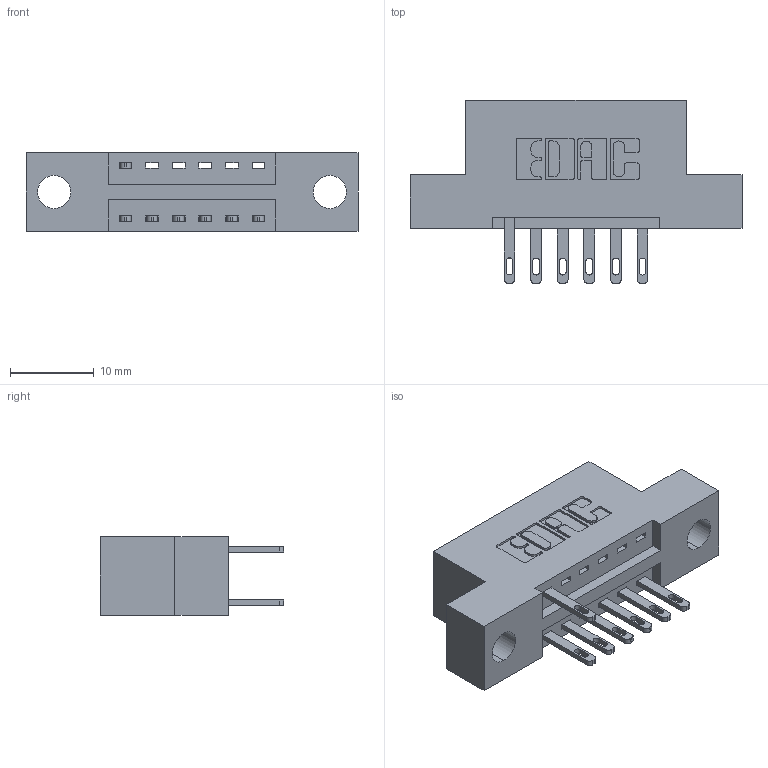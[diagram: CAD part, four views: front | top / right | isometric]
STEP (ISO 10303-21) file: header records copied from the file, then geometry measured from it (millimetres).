
FILE_DESCRIPTION (( 'STEP AP203' ), '1' );
FILE_NAME ('346-012-500-204.STEP', '2018-08-19T21:36:17', ( '' ), ( '' ), 'SwSTEP 2.0', 'SolidWorks 2016', '' );
FILE_SCHEMA (( 'CONFIG_CONTROL_DESIGN' ));
Length unit declared in the file: inch
Products named in the file (3): 346 Part_Flush Mounting Lugs - 0.156 Dia-TH; 345-292-001_345-293-100; 346-012-500-204
Assembly tree (8 placements, depth 2):
  346-012-500-204
    346 Part_Flush Mounting Lugs - 0.156 Dia-TH
    345-292-001_345-293-100  x7
Bounding box: 39.62 x 21.84 x 9.4 mm (x, y, z)
Volume: 3472.8 mm3; surface area: 3834.9 mm2
Topology: 8 solids, 8 shells, 488 faces, 1463 edges, 974 vertices
Faces by surface type: plane 304, cylinder 184
Entity records: 8535 total; most frequent: CARTESIAN_POINT 1475, ORIENTED_EDGE 1414, DIRECTION 1349, EDGE_CURVE 707, VECTOR 547, LINE 547, VERTEX_POINT 470, AXIS2_PLACEMENT_3D 401
